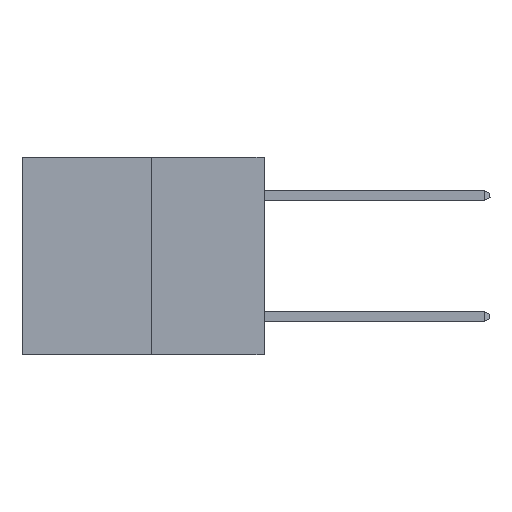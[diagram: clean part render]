
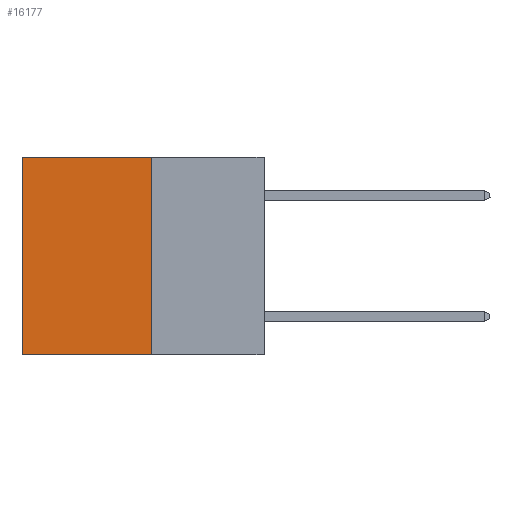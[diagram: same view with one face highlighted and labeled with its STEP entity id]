
A CAD part, left-side view. The second image highlights one B-rep face of the part: STEP entity #16177.
In plain terms, the highlighted planar face has unit normal (-1, 0, 0).
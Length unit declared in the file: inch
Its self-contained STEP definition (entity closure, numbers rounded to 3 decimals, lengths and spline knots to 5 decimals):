
#1109 = VECTOR ( 'NONE', #20517, 39.37008 ) ;
#1616 = EDGE_CURVE ( 'NONE', #5209, #23538, #15817, .T. ) ;
#1736 = VERTEX_POINT ( 'NONE', #3308 ) ;
#1901 = LINE ( 'NONE', #28685, #10049 ) ;
#2130 = EDGE_LOOP ( 'NONE', ( #14902, #2699, #16025, #14537 ) ) ;
#2591 = DIRECTION ( 'NONE',  ( 0., 0., -1. ) ) ;
#2699 = ORIENTED_EDGE ( 'NONE', *, *, #28189, .F. ) ;
#3251 = VECTOR ( 'NONE', #16555, 39.37008 ) ;
#3308 = CARTESIAN_POINT ( 'NONE',  ( 0.3165, 0.6, 0. ) ) ;
#3757 = CARTESIAN_POINT ( 'NONE',  ( 0.3165, 0.28, -0.49 ) ) ;
#4003 = DIRECTION ( 'NONE',  ( 0., 0., -1. ) ) ;
#5209 = VERTEX_POINT ( 'NONE', #25214 ) ;
#5280 = FACE_OUTER_BOUND ( 'NONE', #2130, .T. ) ;
#10049 = VECTOR ( 'NONE', #30626, 39.37008 ) ;
#10841 = LINE ( 'NONE', #25979, #12336 ) ;
#11458 = LINE ( 'NONE', #3757, #1109 ) ;
#11538 = VERTEX_POINT ( 'NONE', #18023 ) ;
#12336 = VECTOR ( 'NONE', #2591, 39.37008 ) ;
#13903 = DIRECTION ( 'NONE',  ( 1., 0., 0. ) ) ;
#14537 = ORIENTED_EDGE ( 'NONE', *, *, #16627, .T. ) ;
#14902 = ORIENTED_EDGE ( 'NONE', *, *, #26353, .T. ) ;
#15817 = LINE ( 'NONE', #26405, #3251 ) ;
#16025 = ORIENTED_EDGE ( 'NONE', *, *, #1616, .F. ) ;
#16094 = CARTESIAN_POINT ( 'NONE',  ( 0.3165, 0.28, -0.49 ) ) ;
#16177 = ADVANCED_FACE ( 'NONE', ( #5280 ), #30288, .F. ) ;
#16555 = DIRECTION ( 'NONE',  ( 0., 0., -1. ) ) ;
#16627 = EDGE_CURVE ( 'NONE', #5209, #1736, #1901, .T. ) ;
#18023 = CARTESIAN_POINT ( 'NONE',  ( 0.3165, 0.6, -0.49 ) ) ;
#18277 = AXIS2_PLACEMENT_3D ( 'NONE', #16094, #13903, #4003 ) ;
#20517 = DIRECTION ( 'NONE',  ( 0., 1., 0. ) ) ;
#21464 = CARTESIAN_POINT ( 'NONE',  ( 0.3165, 0.28, -0.49 ) ) ;
#23538 = VERTEX_POINT ( 'NONE', #21464 ) ;
#25214 = CARTESIAN_POINT ( 'NONE',  ( 0.3165, 0.28, 0. ) ) ;
#25979 = CARTESIAN_POINT ( 'NONE',  ( 0.3165, 0.6, -0.49 ) ) ;
#26353 = EDGE_CURVE ( 'NONE', #1736, #11538, #10841, .T. ) ;
#26405 = CARTESIAN_POINT ( 'NONE',  ( 0.3165, 0.28, -0.49 ) ) ;
#28189 = EDGE_CURVE ( 'NONE', #23538, #11538, #11458, .T. ) ;
#28685 = CARTESIAN_POINT ( 'NONE',  ( 0.3165, 0.28, 0. ) ) ;
#30288 = PLANE ( 'NONE',  #18277 ) ;
#30626 = DIRECTION ( 'NONE',  ( 0., 1., 0. ) ) ;
